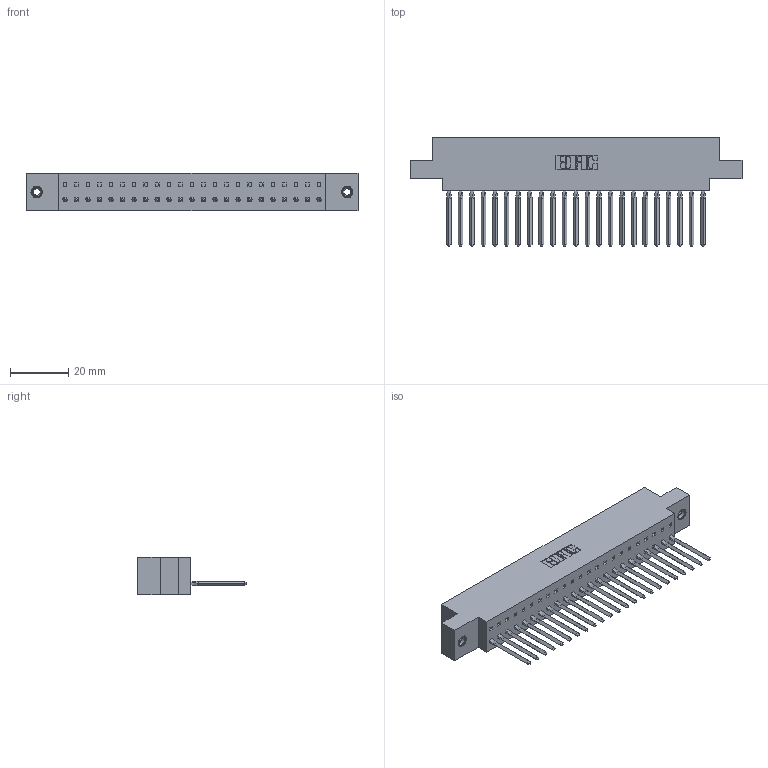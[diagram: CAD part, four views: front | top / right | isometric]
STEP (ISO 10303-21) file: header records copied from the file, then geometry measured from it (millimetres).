
FILE_DESCRIPTION (( 'STEP AP203' ), '1' );
FILE_NAME ('317-023-541-608.STEP', '2020-02-27T17:48:58', ( '' ), ( '' ), 'SwSTEP 2.0', 'SolidWorks 2016', '' );
FILE_SCHEMA (( 'CONFIG_CONTROL_DESIGN' ));
Length unit declared in the file: inch
Products named in the file (4): 345-250-001_345-250-003-102; 317 Part_.156 Dia - TI; 317-290-002_541; 317-023-541-608
Assembly tree (26 placements, depth 2):
  317-023-541-608
    317 Part_.156 Dia - TI
    317-290-002_541  x23
    345-250-001_345-250-003-102  x2
Bounding box: 113.84 x 37.34 x 12.7 mm (x, y, z)
Volume: 17870.7 mm3; surface area: 24640.6 mm2
Topology: 26 solids, 26 shells, 3658 faces, 10393 edges, 6752 vertices
Faces by surface type: plane 2942, cylinder 608, bspline 92, cone 12, torus 4
Entity records: 37895 total; most frequent: CARTESIAN_POINT 7337, ORIENTED_EDGE 6606, DIRECTION 5455, EDGE_CURVE 3303, LINE 2919, VECTOR 2919, VERTEX_POINT 2190, AXIS2_PLACEMENT_3D 1268
